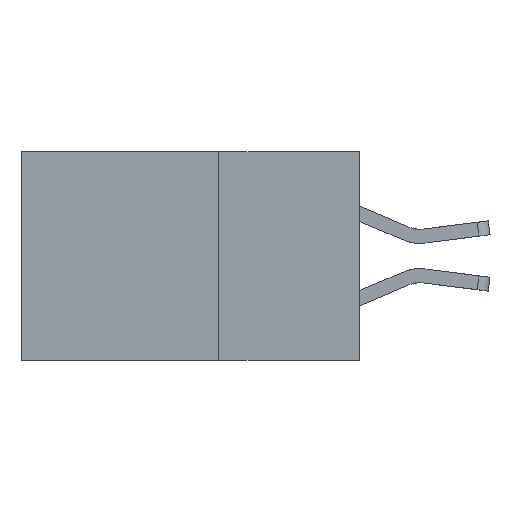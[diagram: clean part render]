
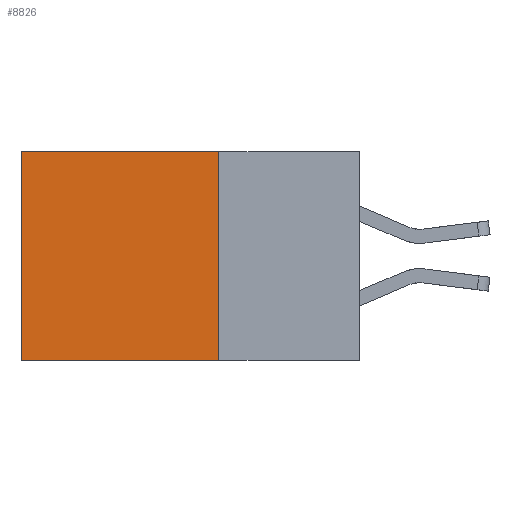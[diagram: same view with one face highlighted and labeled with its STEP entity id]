
A CAD part, left-side view. The second image highlights one B-rep face of the part: STEP entity #8826.
In plain terms, the highlighted planar face has unit normal (-1, 0, 0).
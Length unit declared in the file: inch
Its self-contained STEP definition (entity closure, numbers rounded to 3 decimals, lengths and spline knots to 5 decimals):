
#634 = DIRECTION ( 'NONE',  ( 0., 1., 0. ) ) ;
#936 = ORIENTED_EDGE ( 'NONE', *, *, #2967, .T. ) ;
#973 = EDGE_CURVE ( 'NONE', #1875, #10955, #11316, .T. ) ;
#1875 = VERTEX_POINT ( 'NONE', #7473 ) ;
#1923 = CARTESIAN_POINT ( 'NONE',  ( 0.2875, 0.6, 0. ) ) ;
#2115 = ORIENTED_EDGE ( 'NONE', *, *, #4772, .F. ) ;
#2470 = ORIENTED_EDGE ( 'NONE', *, *, #973, .F. ) ;
#2627 = VECTOR ( 'NONE', #10058, 39.37008 ) ;
#2933 = VERTEX_POINT ( 'NONE', #9793 ) ;
#2967 = EDGE_CURVE ( 'NONE', #2933, #6180, #5371, .T. ) ;
#3768 = AXIS2_PLACEMENT_3D ( 'NONE', #7664, #4499, #11640 ) ;
#3977 = DIRECTION ( 'NONE',  ( 0., 0., -1. ) ) ;
#4499 = DIRECTION ( 'NONE',  ( 1., 0., 0. ) ) ;
#4519 = LINE ( 'NONE', #1923, #11701 ) ;
#4772 = EDGE_CURVE ( 'NONE', #2933, #1875, #9428, .T. ) ;
#5261 = EDGE_LOOP ( 'NONE', ( #7228, #2470, #2115, #936 ) ) ;
#5341 = CARTESIAN_POINT ( 'NONE',  ( 0.2875, 0.6, 0. ) ) ;
#5371 = LINE ( 'NONE', #5604, #6612 ) ;
#5604 = CARTESIAN_POINT ( 'NONE',  ( 0.2875, 0.25, 0. ) ) ;
#5885 = CARTESIAN_POINT ( 'NONE',  ( 0.2875, 0.25, 0. ) ) ;
#6110 = CARTESIAN_POINT ( 'NONE',  ( 0.2875, 0.25, -0.37 ) ) ;
#6180 = VERTEX_POINT ( 'NONE', #5341 ) ;
#6603 = EDGE_CURVE ( 'NONE', #6180, #10955, #4519, .T. ) ;
#6612 = VECTOR ( 'NONE', #634, 39.37008 ) ;
#7154 = FACE_OUTER_BOUND ( 'NONE', #5261, .T. ) ;
#7228 = ORIENTED_EDGE ( 'NONE', *, *, #6603, .T. ) ;
#7473 = CARTESIAN_POINT ( 'NONE',  ( 0.2875, 0.25, -0.37 ) ) ;
#7664 = CARTESIAN_POINT ( 'NONE',  ( 0.2875, 0.25, 0. ) ) ;
#8826 = ADVANCED_FACE ( 'NONE', ( #7154 ), #9663, .F. ) ;
#9066 = DIRECTION ( 'NONE',  ( 0., 1., 0. ) ) ;
#9428 = LINE ( 'NONE', #5885, #2627 ) ;
#9663 = PLANE ( 'NONE',  #3768 ) ;
#9793 = CARTESIAN_POINT ( 'NONE',  ( 0.2875, 0.25, 0. ) ) ;
#10058 = DIRECTION ( 'NONE',  ( 0., 0., -1. ) ) ;
#10955 = VERTEX_POINT ( 'NONE', #12240 ) ;
#11316 = LINE ( 'NONE', #6110, #12273 ) ;
#11640 = DIRECTION ( 'NONE',  ( 0., 0., -1. ) ) ;
#11701 = VECTOR ( 'NONE', #3977, 39.37008 ) ;
#12240 = CARTESIAN_POINT ( 'NONE',  ( 0.2875, 0.6, -0.37 ) ) ;
#12273 = VECTOR ( 'NONE', #9066, 39.37008 ) ;
